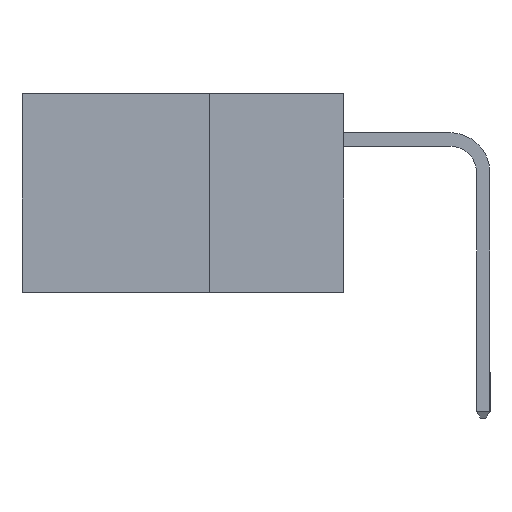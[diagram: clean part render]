
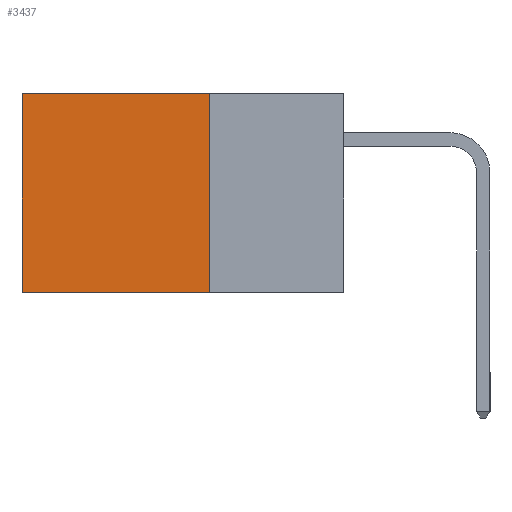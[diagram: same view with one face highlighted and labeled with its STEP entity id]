
A CAD part, left-side view. The second image highlights one B-rep face of the part: STEP entity #3437.
In plain terms, the highlighted planar face has unit normal (-1, 0, 0).
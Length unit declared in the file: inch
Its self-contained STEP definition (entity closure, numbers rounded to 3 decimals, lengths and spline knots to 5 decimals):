
#537 = DIRECTION ( 'NONE',  ( 0., 0., -1. ) ) ;
#619 = LINE ( 'NONE', #18967, #16596 ) ;
#877 = LINE ( 'NONE', #2343, #15552 ) ;
#2343 = CARTESIAN_POINT ( 'NONE',  ( 0.298, 0.25, -0.37 ) ) ;
#2511 = CARTESIAN_POINT ( 'NONE',  ( 0.298, 0.25, 0. ) ) ;
#3437 = ADVANCED_FACE ( 'NONE', ( #3948 ), #12981, .F. ) ;
#3659 = CARTESIAN_POINT ( 'NONE',  ( 0.298, 0.25, 0. ) ) ;
#3721 = CARTESIAN_POINT ( 'NONE',  ( 0.298, 0.6, 0. ) ) ;
#3773 = ORIENTED_EDGE ( 'NONE', *, *, #15509, .T. ) ;
#3948 = FACE_OUTER_BOUND ( 'NONE', #16616, .T. ) ;
#6161 = VERTEX_POINT ( 'NONE', #22041 ) ;
#6519 = DIRECTION ( 'NONE',  ( 0., 0., -1. ) ) ;
#6711 = DIRECTION ( 'NONE',  ( 1., 0., 0. ) ) ;
#7429 = EDGE_CURVE ( 'NONE', #19795, #13409, #16759, .T. ) ;
#8134 = DIRECTION ( 'NONE',  ( 0., 1., 0. ) ) ;
#8608 = DIRECTION ( 'NONE',  ( 0., 0., -1. ) ) ;
#8828 = CARTESIAN_POINT ( 'NONE',  ( 0.298, 0.25, 0. ) ) ;
#9250 = VECTOR ( 'NONE', #8134, 39.37008 ) ;
#9503 = VERTEX_POINT ( 'NONE', #26536 ) ;
#9907 = EDGE_CURVE ( 'NONE', #19795, #9503, #19380, .T. ) ;
#10733 = ORIENTED_EDGE ( 'NONE', *, *, #9907, .F. ) ;
#12631 = ORIENTED_EDGE ( 'NONE', *, *, #7429, .T. ) ;
#12835 = DIRECTION ( 'NONE',  ( 0., 1., 0. ) ) ;
#12981 = PLANE ( 'NONE',  #15806 ) ;
#13409 = VERTEX_POINT ( 'NONE', #3721 ) ;
#15509 = EDGE_CURVE ( 'NONE', #13409, #6161, #619, .T. ) ;
#15552 = VECTOR ( 'NONE', #12835, 39.37008 ) ;
#15806 = AXIS2_PLACEMENT_3D ( 'NONE', #18892, #6711, #8608 ) ;
#16596 = VECTOR ( 'NONE', #6519, 39.37008 ) ;
#16616 = EDGE_LOOP ( 'NONE', ( #3773, #20640, #10733, #12631 ) ) ;
#16759 = LINE ( 'NONE', #3659, #9250 ) ;
#18892 = CARTESIAN_POINT ( 'NONE',  ( 0.298, 0.25, 0. ) ) ;
#18967 = CARTESIAN_POINT ( 'NONE',  ( 0.298, 0.6, 0. ) ) ;
#19380 = LINE ( 'NONE', #8828, #21991 ) ;
#19795 = VERTEX_POINT ( 'NONE', #2511 ) ;
#20640 = ORIENTED_EDGE ( 'NONE', *, *, #26100, .F. ) ;
#21991 = VECTOR ( 'NONE', #537, 39.37008 ) ;
#22041 = CARTESIAN_POINT ( 'NONE',  ( 0.298, 0.6, -0.37 ) ) ;
#26100 = EDGE_CURVE ( 'NONE', #9503, #6161, #877, .T. ) ;
#26536 = CARTESIAN_POINT ( 'NONE',  ( 0.298, 0.25, -0.37 ) ) ;
